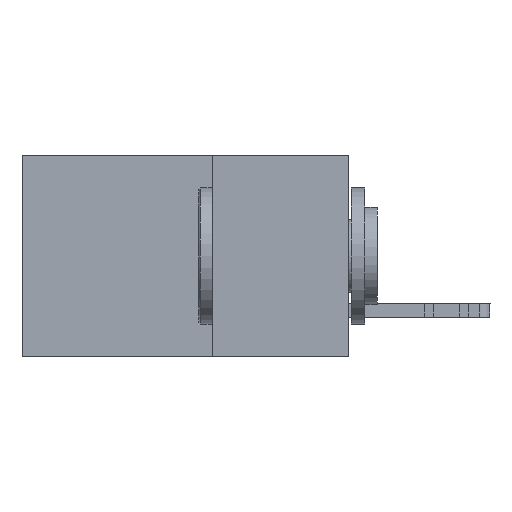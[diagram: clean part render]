
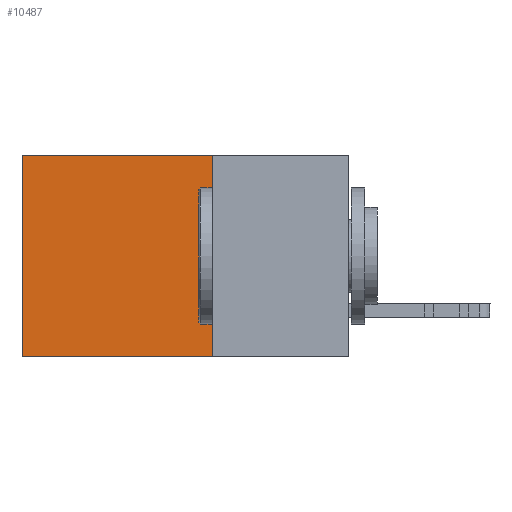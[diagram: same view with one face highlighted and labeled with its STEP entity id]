
A CAD part, left-side view. The second image highlights one B-rep face of the part: STEP entity #10487.
In plain terms, the highlighted planar face has unit normal (-1, 0, 0).
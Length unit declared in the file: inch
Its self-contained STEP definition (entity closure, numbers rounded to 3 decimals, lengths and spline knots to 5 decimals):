
#529 = VECTOR ( 'NONE', #1404, 39.37008 ) ;
#674 = CARTESIAN_POINT ( 'NONE',  ( 0.2615, 0.6, -0.37 ) ) ;
#808 = VECTOR ( 'NONE', #15994, 39.37008 ) ;
#982 = PLANE ( 'NONE',  #8905 ) ;
#1102 = ORIENTED_EDGE ( 'NONE', *, *, #9486, .F. ) ;
#1404 = DIRECTION ( 'NONE',  ( 0., 1., 0. ) ) ;
#1594 = CARTESIAN_POINT ( 'NONE',  ( 0.2615, 0.25, -0.37 ) ) ;
#1797 = CARTESIAN_POINT ( 'NONE',  ( 0.2615, 0.25, 0. ) ) ;
#1880 = ORIENTED_EDGE ( 'NONE', *, *, #18066, .F. ) ;
#2426 = VERTEX_POINT ( 'NONE', #1594 ) ;
#2775 = VECTOR ( 'NONE', #8111, 39.37008 ) ;
#4151 = VERTEX_POINT ( 'NONE', #1797 ) ;
#5464 = LINE ( 'NONE', #14242, #9538 ) ;
#6041 = EDGE_CURVE ( 'NONE', #11036, #9737, #5464, .T. ) ;
#6603 = CARTESIAN_POINT ( 'NONE',  ( 0.2615, 0.6, 0. ) ) ;
#8111 = DIRECTION ( 'NONE',  ( 0., 1., 0. ) ) ;
#8905 = AXIS2_PLACEMENT_3D ( 'NONE', #14953, #20597, #16914 ) ;
#9486 = EDGE_CURVE ( 'NONE', #2426, #9737, #11219, .T. ) ;
#9538 = VECTOR ( 'NONE', #19506, 39.37008 ) ;
#9737 = VERTEX_POINT ( 'NONE', #674 ) ;
#10487 = ADVANCED_FACE ( 'NONE', ( #17849 ), #982, .F. ) ;
#11036 = VERTEX_POINT ( 'NONE', #6603 ) ;
#11219 = LINE ( 'NONE', #17291, #529 ) ;
#12767 = EDGE_CURVE ( 'NONE', #4151, #11036, #23548, .T. ) ;
#13734 = ORIENTED_EDGE ( 'NONE', *, *, #6041, .T. ) ;
#14030 = CARTESIAN_POINT ( 'NONE',  ( 0.2615, 0.25, -0.37 ) ) ;
#14242 = CARTESIAN_POINT ( 'NONE',  ( 0.2615, 0.6, -0.37 ) ) ;
#14953 = CARTESIAN_POINT ( 'NONE',  ( 0.2615, 0.25, -0.37 ) ) ;
#15994 = DIRECTION ( 'NONE',  ( 0., 0., -1. ) ) ;
#16914 = DIRECTION ( 'NONE',  ( 0., 0., -1. ) ) ;
#17291 = CARTESIAN_POINT ( 'NONE',  ( 0.2615, 0.25, -0.37 ) ) ;
#17849 = FACE_OUTER_BOUND ( 'NONE', #25127, .T. ) ;
#18066 = EDGE_CURVE ( 'NONE', #4151, #2426, #22298, .T. ) ;
#19506 = DIRECTION ( 'NONE',  ( 0., 0., -1. ) ) ;
#19765 = CARTESIAN_POINT ( 'NONE',  ( 0.2615, 0.25, 0. ) ) ;
#20597 = DIRECTION ( 'NONE',  ( 1., 0., 0. ) ) ;
#22298 = LINE ( 'NONE', #14030, #808 ) ;
#23441 = ORIENTED_EDGE ( 'NONE', *, *, #12767, .T. ) ;
#23548 = LINE ( 'NONE', #19765, #2775 ) ;
#25127 = EDGE_LOOP ( 'NONE', ( #13734, #1102, #1880, #23441 ) ) ;
